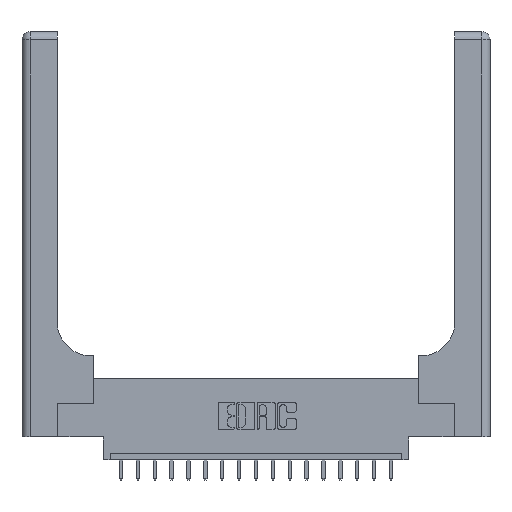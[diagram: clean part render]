
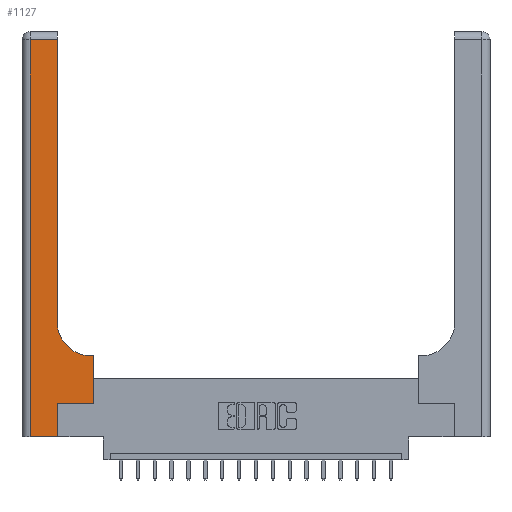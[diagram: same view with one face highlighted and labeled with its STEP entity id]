
A CAD part, top view. The second image highlights one B-rep face of the part: STEP entity #1127.
In plain terms, the highlighted planar face has unit normal (0, 0, 1).
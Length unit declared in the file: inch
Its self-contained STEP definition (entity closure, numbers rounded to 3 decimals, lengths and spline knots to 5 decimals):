
#274 = CARTESIAN_POINT ( 'NONE',  ( 0.265, 0., 0.37 ) ) ;
#432 = CARTESIAN_POINT ( 'NONE',  ( 0.26, 2.94, 0.37 ) ) ;
#510 = VERTEX_POINT ( 'NONE', #3501 ) ;
#766 = CARTESIAN_POINT ( 'NONE',  ( 0.528, 0.25, 0.37 ) ) ;
#791 = DIRECTION ( 'NONE',  ( 0., -1., 0. ) ) ;
#1083 = DIRECTION ( 'NONE',  ( -1., 0., 0. ) ) ;
#1127 = ADVANCED_FACE ( 'NONE', ( #12907 ), #3966, .F. ) ;
#2795 = ORIENTED_EDGE ( 'NONE', *, *, #17204, .T. ) ;
#2824 = DIRECTION ( 'NONE',  ( -1., 0., 0. ) ) ;
#3501 = CARTESIAN_POINT ( 'NONE',  ( 0.51, 0.6, 0.37 ) ) ;
#3526 = ORIENTED_EDGE ( 'NONE', *, *, #7734, .T. ) ;
#3879 = LINE ( 'NONE', #12920, #16979 ) ;
#3966 = PLANE ( 'NONE',  #9202 ) ;
#4047 = VERTEX_POINT ( 'NONE', #7062 ) ;
#4864 = DIRECTION ( 'NONE',  ( 1., 0., 0. ) ) ;
#4909 = VECTOR ( 'NONE', #6545, 39.37008 ) ;
#5416 = LINE ( 'NONE', #7107, #6376 ) ;
#5694 = CARTESIAN_POINT ( 'NONE',  ( 0., 0., 0.37 ) ) ;
#5892 = VERTEX_POINT ( 'NONE', #274 ) ;
#6053 = LINE ( 'NONE', #14732, #15519 ) ;
#6376 = VECTOR ( 'NONE', #13178, 39.37008 ) ;
#6545 = DIRECTION ( 'NONE',  ( 0., 1., 0. ) ) ;
#6737 = LINE ( 'NONE', #766, #4909 ) ;
#6987 = EDGE_CURVE ( 'NONE', #19678, #10202, #6053, .T. ) ;
#7062 = CARTESIAN_POINT ( 'NONE',  ( 0.265, 0.25, 0.37 ) ) ;
#7107 = CARTESIAN_POINT ( 'NONE',  ( 0.26, 3., 0.37 ) ) ;
#7620 = VERTEX_POINT ( 'NONE', #11679 ) ;
#7718 = EDGE_CURVE ( 'NONE', #510, #12932, #18662, .T. ) ;
#7734 = EDGE_CURVE ( 'NONE', #8431, #510, #17769, .T. ) ;
#7838 = CARTESIAN_POINT ( 'NONE',  ( 0.265, 0.25, 0.37 ) ) ;
#8431 = VERTEX_POINT ( 'NONE', #17407 ) ;
#8776 = LINE ( 'NONE', #5694, #17446 ) ;
#9048 = ORIENTED_EDGE ( 'NONE', *, *, #12217, .T. ) ;
#9202 = AXIS2_PLACEMENT_3D ( 'NONE', #9831, #15909, #15814 ) ;
#9378 = EDGE_CURVE ( 'NONE', #7620, #5892, #8776, .T. ) ;
#9399 = EDGE_CURVE ( 'NONE', #5892, #4047, #14762, .T. ) ;
#9754 = VECTOR ( 'NONE', #2824, 39.37008 ) ;
#9758 = ORIENTED_EDGE ( 'NONE', *, *, #9399, .T. ) ;
#9831 = CARTESIAN_POINT ( 'NONE',  ( 0., 3., 0.37 ) ) ;
#10202 = VERTEX_POINT ( 'NONE', #19391 ) ;
#10295 = DIRECTION ( 'NONE',  ( 0., 0., -1. ) ) ;
#10296 = VERTEX_POINT ( 'NONE', #13013 ) ;
#10528 = LINE ( 'NONE', #7838, #11770 ) ;
#11216 = ORIENTED_EDGE ( 'NONE', *, *, #17650, .T. ) ;
#11679 = CARTESIAN_POINT ( 'NONE',  ( 0.06, 0., 0.37 ) ) ;
#11701 = EDGE_CURVE ( 'NONE', #4047, #10296, #10528, .T. ) ;
#11770 = VECTOR ( 'NONE', #4864, 39.37008 ) ;
#12217 = EDGE_CURVE ( 'NONE', #12932, #19678, #5416, .T. ) ;
#12349 = ORIENTED_EDGE ( 'NONE', *, *, #11701, .T. ) ;
#12907 = FACE_OUTER_BOUND ( 'NONE', #16171, .T. ) ;
#12920 = CARTESIAN_POINT ( 'NONE',  ( 0.06, 3., 0.37 ) ) ;
#12932 = VERTEX_POINT ( 'NONE', #18302 ) ;
#12933 = AXIS2_PLACEMENT_3D ( 'NONE', #17669, #10295, #17968 ) ;
#12946 = ORIENTED_EDGE ( 'NONE', *, *, #7718, .T. ) ;
#13013 = CARTESIAN_POINT ( 'NONE',  ( 0.528, 0.25, 0.37 ) ) ;
#13057 = CARTESIAN_POINT ( 'NONE',  ( 0.265, 0., 0.37 ) ) ;
#13058 = ORIENTED_EDGE ( 'NONE', *, *, #6987, .T. ) ;
#13178 = DIRECTION ( 'NONE',  ( 0., 1., 0. ) ) ;
#13254 = DIRECTION ( 'NONE',  ( 0., 1., 0. ) ) ;
#13700 = ORIENTED_EDGE ( 'NONE', *, *, #9378, .T. ) ;
#14572 = VECTOR ( 'NONE', #13254, 39.37008 ) ;
#14732 = CARTESIAN_POINT ( 'NONE',  ( 0., 2.94, 0.37 ) ) ;
#14762 = LINE ( 'NONE', #13057, #14572 ) ;
#14854 = DIRECTION ( 'NONE',  ( 1., 0., 0. ) ) ;
#15519 = VECTOR ( 'NONE', #1083, 39.37008 ) ;
#15814 = DIRECTION ( 'NONE',  ( -1., 0., 0. ) ) ;
#15909 = DIRECTION ( 'NONE',  ( 0., 0., -1. ) ) ;
#16171 = EDGE_LOOP ( 'NONE', ( #9048, #13058, #2795, #13700, #9758, #12349, #11216, #3526, #12946 ) ) ;
#16471 = CARTESIAN_POINT ( 'NONE',  ( 0.26, 0.6, 0.37 ) ) ;
#16979 = VECTOR ( 'NONE', #791, 39.37008 ) ;
#17204 = EDGE_CURVE ( 'NONE', #10202, #7620, #3879, .T. ) ;
#17407 = CARTESIAN_POINT ( 'NONE',  ( 0.528, 0.6, 0.37 ) ) ;
#17446 = VECTOR ( 'NONE', #14854, 39.37008 ) ;
#17650 = EDGE_CURVE ( 'NONE', #10296, #8431, #6737, .T. ) ;
#17669 = CARTESIAN_POINT ( 'NONE',  ( 0.51, 0.85, 0.37 ) ) ;
#17769 = LINE ( 'NONE', #16471, #9754 ) ;
#17968 = DIRECTION ( 'NONE',  ( 1., 0., 0. ) ) ;
#18302 = CARTESIAN_POINT ( 'NONE',  ( 0.26, 0.85, 0.37 ) ) ;
#18662 = CIRCLE ( 'NONE', #12933, 0.25 ) ;
#19391 = CARTESIAN_POINT ( 'NONE',  ( 0.06, 2.94, 0.37 ) ) ;
#19678 = VERTEX_POINT ( 'NONE', #432 ) ;
